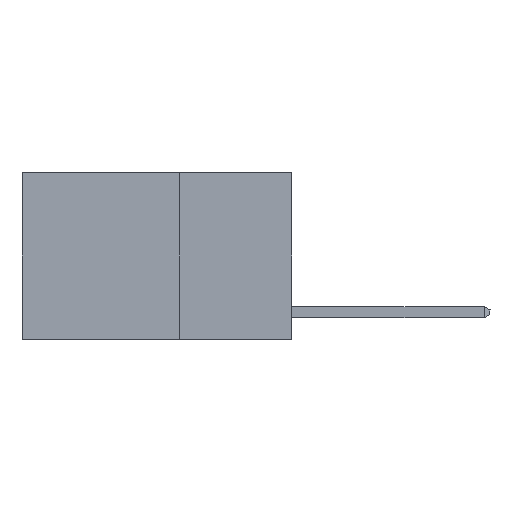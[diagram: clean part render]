
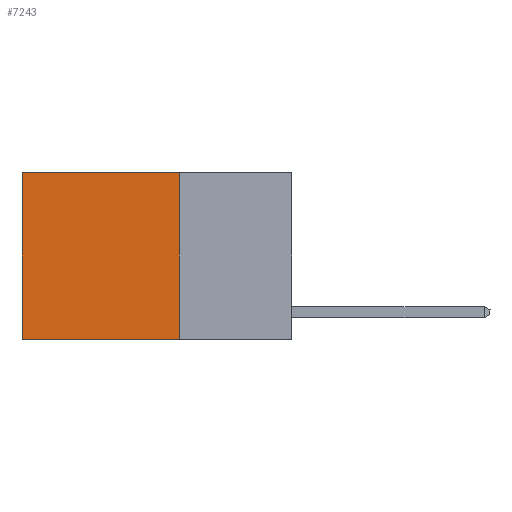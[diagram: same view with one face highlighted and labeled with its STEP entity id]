
A CAD part, left-side view. The second image highlights one B-rep face of the part: STEP entity #7243.
In plain terms, the highlighted planar face has unit normal (-1, 0, 0).
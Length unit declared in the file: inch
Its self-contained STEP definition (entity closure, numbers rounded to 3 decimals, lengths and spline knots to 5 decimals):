
#62 = CARTESIAN_POINT ( 'NONE',  ( 0.2625, 0.25, 0. ) ) ;
#361 = LINE ( 'NONE', #62, #5742 ) ;
#709 = EDGE_CURVE ( 'NONE', #22155, #834, #17526, .T. ) ;
#833 = CARTESIAN_POINT ( 'NONE',  ( 0.2625, 0.6, 0. ) ) ;
#834 = VERTEX_POINT ( 'NONE', #2170 ) ;
#1016 = DIRECTION ( 'NONE',  ( 0., 0., -1. ) ) ;
#1180 = ORIENTED_EDGE ( 'NONE', *, *, #1424, .T. ) ;
#1424 = EDGE_CURVE ( 'NONE', #6213, #834, #21392, .T. ) ;
#2170 = CARTESIAN_POINT ( 'NONE',  ( 0.2625, 0.6, -0.37 ) ) ;
#2525 = AXIS2_PLACEMENT_3D ( 'NONE', #12936, #18289, #7606 ) ;
#3680 = EDGE_CURVE ( 'NONE', #20130, #6213, #23061, .T. ) ;
#4043 = EDGE_CURVE ( 'NONE', #20130, #22155, #361, .T. ) ;
#5647 = EDGE_LOOP ( 'NONE', ( #1180, #16302, #16951, #10674 ) ) ;
#5742 = VECTOR ( 'NONE', #7357, 39.37008 ) ;
#5762 = PLANE ( 'NONE',  #2525 ) ;
#6213 = VERTEX_POINT ( 'NONE', #11885 ) ;
#7243 = ADVANCED_FACE ( 'NONE', ( #17080 ), #5762, .F. ) ;
#7357 = DIRECTION ( 'NONE',  ( 0., 0., -1. ) ) ;
#7606 = DIRECTION ( 'NONE',  ( 0., 0., -1. ) ) ;
#8043 = CARTESIAN_POINT ( 'NONE',  ( 0.2625, 0.25, 0. ) ) ;
#8898 = VECTOR ( 'NONE', #18844, 39.37008 ) ;
#10674 = ORIENTED_EDGE ( 'NONE', *, *, #3680, .T. ) ;
#11885 = CARTESIAN_POINT ( 'NONE',  ( 0.2625, 0.6, 0. ) ) ;
#12936 = CARTESIAN_POINT ( 'NONE',  ( 0.2625, 0.25, 0. ) ) ;
#13556 = CARTESIAN_POINT ( 'NONE',  ( 0.2625, 0.25, 0. ) ) ;
#14366 = DIRECTION ( 'NONE',  ( 0., 1., 0. ) ) ;
#15018 = CARTESIAN_POINT ( 'NONE',  ( 0.2625, 0.25, -0.37 ) ) ;
#16302 = ORIENTED_EDGE ( 'NONE', *, *, #709, .F. ) ;
#16951 = ORIENTED_EDGE ( 'NONE', *, *, #4043, .F. ) ;
#17080 = FACE_OUTER_BOUND ( 'NONE', #5647, .T. ) ;
#17526 = LINE ( 'NONE', #15018, #18092 ) ;
#18092 = VECTOR ( 'NONE', #14366, 39.37008 ) ;
#18289 = DIRECTION ( 'NONE',  ( 1., 0., 0. ) ) ;
#18844 = DIRECTION ( 'NONE',  ( 0., 1., 0. ) ) ;
#20130 = VERTEX_POINT ( 'NONE', #8043 ) ;
#20846 = VECTOR ( 'NONE', #1016, 39.37008 ) ;
#21392 = LINE ( 'NONE', #833, #20846 ) ;
#22155 = VERTEX_POINT ( 'NONE', #22398 ) ;
#22398 = CARTESIAN_POINT ( 'NONE',  ( 0.2625, 0.25, -0.37 ) ) ;
#23061 = LINE ( 'NONE', #13556, #8898 ) ;
